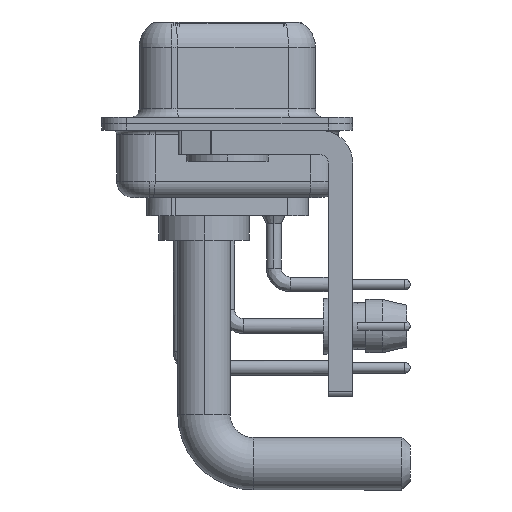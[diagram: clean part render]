
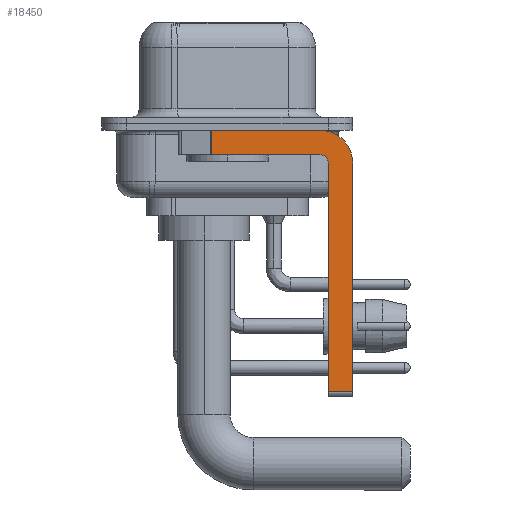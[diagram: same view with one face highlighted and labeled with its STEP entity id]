
A CAD part, left-side view. The second image highlights one B-rep face of the part: STEP entity #18450.
In plain terms, the highlighted planar face has unit normal (-1, 0, 0).
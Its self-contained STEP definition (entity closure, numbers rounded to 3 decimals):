
#1854 = LINE ( 'NONE', #4790, #23245 ) ;
#3134 = ORIENTED_EDGE ( 'NONE', *, *, #9265, .F. ) ;
#3614 = VECTOR ( 'NONE', #17416, 1000. ) ;
#4435 = EDGE_LOOP ( 'NONE', ( #3134, #24730, #25577, #28030, #18307, #16980, #14537, #6926 ) ) ;
#4516 = FACE_OUTER_BOUND ( 'NONE', #4435, .T. ) ;
#4680 = VERTEX_POINT ( 'NONE', #5149 ) ;
#4790 = CARTESIAN_POINT ( 'NONE',  ( -2.9, -7.65, -2.4 ) ) ;
#4981 = DIRECTION ( 'NONE',  ( 0., 0., -1. ) ) ;
#5149 = CARTESIAN_POINT ( 'NONE',  ( -2.9, 0.978, -1.9 ) ) ;
#5166 = AXIS2_PLACEMENT_3D ( 'NONE', #12307, #34901, #9734 ) ;
#5931 = DIRECTION ( 'NONE',  ( -1., 0., 0. ) ) ;
#6154 = VERTEX_POINT ( 'NONE', #24163 ) ;
#6224 = AXIS2_PLACEMENT_3D ( 'NONE', #33843, #5931, #17133 ) ;
#6926 = ORIENTED_EDGE ( 'NONE', *, *, #14819, .F. ) ;
#7089 = VERTEX_POINT ( 'NONE', #7973 ) ;
#7973 = CARTESIAN_POINT ( 'NONE',  ( -2.9, -5.65, -0.4 ) ) ;
#8228 = LINE ( 'NONE', #10817, #15015 ) ;
#9174 = CIRCLE ( 'NONE', #6224, 0.5 ) ;
#9265 = EDGE_CURVE ( 'NONE', #15655, #7089, #36024, .T. ) ;
#9729 = VECTOR ( 'NONE', #19250, 1000. ) ;
#9734 = DIRECTION ( 'NONE',  ( 0., 0., -1. ) ) ;
#9777 = DIRECTION ( 'NONE',  ( 0., 0., 1. ) ) ;
#10686 = CARTESIAN_POINT ( 'NONE',  ( -2.9, -5.65, -1.9 ) ) ;
#10817 = CARTESIAN_POINT ( 'NONE',  ( -2.9, -5.65, -1.9 ) ) ;
#11959 = VERTEX_POINT ( 'NONE', #22535 ) ;
#12307 = CARTESIAN_POINT ( 'NONE',  ( -2.9, -5.65, -2.4 ) ) ;
#13164 = EDGE_CURVE ( 'NONE', #35855, #30893, #1854, .T. ) ;
#14327 = LINE ( 'NONE', #31208, #3614 ) ;
#14537 = ORIENTED_EDGE ( 'NONE', *, *, #13164, .F. ) ;
#14819 = EDGE_CURVE ( 'NONE', #7089, #35855, #33320, .T. ) ;
#15015 = VECTOR ( 'NONE', #22188, 1000. ) ;
#15655 = VERTEX_POINT ( 'NONE', #29449 ) ;
#15917 = CARTESIAN_POINT ( 'NONE',  ( -2.9, -5.65, -2.4 ) ) ;
#16458 = AXIS2_PLACEMENT_3D ( 'NONE', #15917, #22134, #27107 ) ;
#16564 = VECTOR ( 'NONE', #9777, 1000. ) ;
#16980 = ORIENTED_EDGE ( 'NONE', *, *, #23769, .T. ) ;
#17133 = DIRECTION ( 'NONE',  ( 0., 0., 1. ) ) ;
#17416 = DIRECTION ( 'NONE',  ( 0., 0., -1. ) ) ;
#18307 = ORIENTED_EDGE ( 'NONE', *, *, #21060, .F. ) ;
#18450 = ADVANCED_FACE ( 'NONE', ( #4516 ), #27637, .F. ) ;
#19185 = EDGE_CURVE ( 'NONE', #15655, #4680, #14327, .T. ) ;
#19250 = DIRECTION ( 'NONE',  ( 0., -1., 0. ) ) ;
#20621 = CARTESIAN_POINT ( 'NONE',  ( -2.9, -6.15, -16.6 ) ) ;
#21060 = EDGE_CURVE ( 'NONE', #6154, #11959, #28685, .T. ) ;
#21265 = VERTEX_POINT ( 'NONE', #10686 ) ;
#22134 = DIRECTION ( 'NONE',  ( 1., 0., 0. ) ) ;
#22188 = DIRECTION ( 'NONE',  ( 0., 1., 0. ) ) ;
#22535 = CARTESIAN_POINT ( 'NONE',  ( -2.9, -6.15, -2.4 ) ) ;
#23245 = VECTOR ( 'NONE', #4981, 1000. ) ;
#23769 = EDGE_CURVE ( 'NONE', #6154, #30893, #32679, .T. ) ;
#23838 = EDGE_CURVE ( 'NONE', #21265, #4680, #8228, .T. ) ;
#24163 = CARTESIAN_POINT ( 'NONE',  ( -2.9, -6.15, -16.35 ) ) ;
#24442 = EDGE_CURVE ( 'NONE', #11959, #21265, #9174, .T. ) ;
#24730 = ORIENTED_EDGE ( 'NONE', *, *, #19185, .T. ) ;
#25549 = CARTESIAN_POINT ( 'NONE',  ( -2.9, -7.65, -2.4 ) ) ;
#25577 = ORIENTED_EDGE ( 'NONE', *, *, #23838, .F. ) ;
#27107 = DIRECTION ( 'NONE',  ( 0., 0., -1. ) ) ;
#27355 = CARTESIAN_POINT ( 'NONE',  ( -2.9, 3., -0.4 ) ) ;
#27637 = PLANE ( 'NONE',  #16458 ) ;
#28030 = ORIENTED_EDGE ( 'NONE', *, *, #24442, .F. ) ;
#28685 = LINE ( 'NONE', #20621, #16564 ) ;
#29193 = CARTESIAN_POINT ( 'NONE',  ( -2.9, -5.65, -16.35 ) ) ;
#29449 = CARTESIAN_POINT ( 'NONE',  ( -2.9, 0.978, -0.4 ) ) ;
#29718 = CARTESIAN_POINT ( 'NONE',  ( -2.9, -7.65, -16.35 ) ) ;
#30012 = VECTOR ( 'NONE', #32698, 1000. ) ;
#30893 = VERTEX_POINT ( 'NONE', #29718 ) ;
#31208 = CARTESIAN_POINT ( 'NONE',  ( -2.9, 0.978, -1.9 ) ) ;
#32679 = LINE ( 'NONE', #29193, #9729 ) ;
#32698 = DIRECTION ( 'NONE',  ( 0., -1., 0. ) ) ;
#33320 = CIRCLE ( 'NONE', #5166, 2. ) ;
#33843 = CARTESIAN_POINT ( 'NONE',  ( -2.9, -5.65, -2.4 ) ) ;
#34901 = DIRECTION ( 'NONE',  ( 1., 0., 0. ) ) ;
#35855 = VERTEX_POINT ( 'NONE', #25549 ) ;
#36024 = LINE ( 'NONE', #27355, #30012 ) ;
